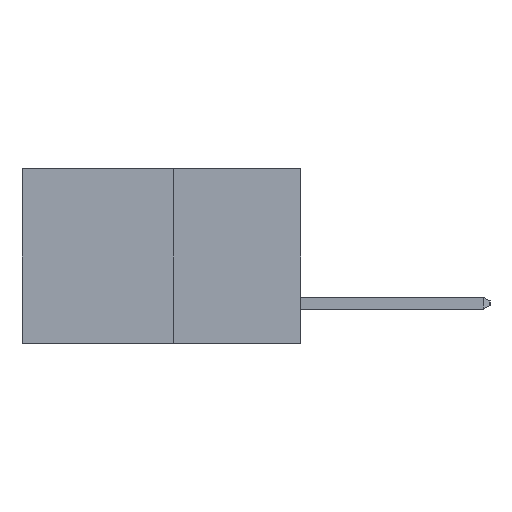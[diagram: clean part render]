
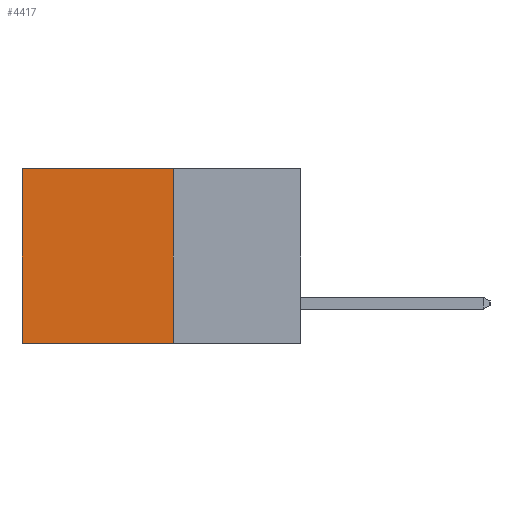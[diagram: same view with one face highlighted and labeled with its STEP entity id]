
A CAD part, left-side view. The second image highlights one B-rep face of the part: STEP entity #4417.
In plain terms, the highlighted planar face has unit normal (-1, 0, 0).
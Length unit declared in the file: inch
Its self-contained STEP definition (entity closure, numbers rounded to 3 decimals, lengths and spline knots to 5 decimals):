
#4 = VERTEX_POINT ( 'NONE', #6772 ) ;
#345 = LINE ( 'NONE', #6931, #3408 ) ;
#367 = CARTESIAN_POINT ( 'NONE',  ( 0.277, 0.27, -0.37 ) ) ;
#1009 = CARTESIAN_POINT ( 'NONE',  ( 0.277, 0.59, -0.37 ) ) ;
#2015 = ORIENTED_EDGE ( 'NONE', *, *, #9717, .F. ) ;
#2124 = LINE ( 'NONE', #2334, #11357 ) ;
#2334 = CARTESIAN_POINT ( 'NONE',  ( 0.277, 0.27, -0.37 ) ) ;
#2669 = EDGE_CURVE ( 'NONE', #5459, #7830, #2124, .T. ) ;
#2677 = PLANE ( 'NONE',  #9552 ) ;
#3334 = DIRECTION ( 'NONE',  ( 0., 0., -1. ) ) ;
#3408 = VECTOR ( 'NONE', #5956, 39.37008 ) ;
#3771 = ORIENTED_EDGE ( 'NONE', *, *, #2669, .F. ) ;
#4417 = ADVANCED_FACE ( 'NONE', ( #11309 ), #2677, .F. ) ;
#4422 = VECTOR ( 'NONE', #10625, 39.37008 ) ;
#4729 = DIRECTION ( 'NONE',  ( 0., 0., -1. ) ) ;
#4837 = VERTEX_POINT ( 'NONE', #1009 ) ;
#5459 = VERTEX_POINT ( 'NONE', #6664 ) ;
#5956 = DIRECTION ( 'NONE',  ( 0., 0., -1. ) ) ;
#6130 = EDGE_CURVE ( 'NONE', #5459, #4, #11535, .T. ) ;
#6463 = CARTESIAN_POINT ( 'NONE',  ( 0.277, 0.27, -0.37 ) ) ;
#6664 = CARTESIAN_POINT ( 'NONE',  ( 0.277, 0.27, 0. ) ) ;
#6772 = CARTESIAN_POINT ( 'NONE',  ( 0.277, 0.59, 0. ) ) ;
#6931 = CARTESIAN_POINT ( 'NONE',  ( 0.277, 0.59, -0.37 ) ) ;
#7064 = DIRECTION ( 'NONE',  ( 1., 0., 0. ) ) ;
#7591 = CARTESIAN_POINT ( 'NONE',  ( 0.277, 0.27, -0.37 ) ) ;
#7830 = VERTEX_POINT ( 'NONE', #367 ) ;
#8368 = ORIENTED_EDGE ( 'NONE', *, *, #6130, .T. ) ;
#8791 = EDGE_CURVE ( 'NONE', #4, #4837, #345, .T. ) ;
#8815 = ORIENTED_EDGE ( 'NONE', *, *, #8791, .T. ) ;
#9286 = VECTOR ( 'NONE', #11901, 39.37008 ) ;
#9552 = AXIS2_PLACEMENT_3D ( 'NONE', #6463, #7064, #3334 ) ;
#9717 = EDGE_CURVE ( 'NONE', #7830, #4837, #11588, .T. ) ;
#10625 = DIRECTION ( 'NONE',  ( 0., 1., 0. ) ) ;
#10635 = CARTESIAN_POINT ( 'NONE',  ( 0.277, 0.27, 0. ) ) ;
#11309 = FACE_OUTER_BOUND ( 'NONE', #11537, .T. ) ;
#11357 = VECTOR ( 'NONE', #4729, 39.37008 ) ;
#11535 = LINE ( 'NONE', #10635, #4422 ) ;
#11537 = EDGE_LOOP ( 'NONE', ( #8815, #2015, #3771, #8368 ) ) ;
#11588 = LINE ( 'NONE', #7591, #9286 ) ;
#11901 = DIRECTION ( 'NONE',  ( 0., 1., 0. ) ) ;
